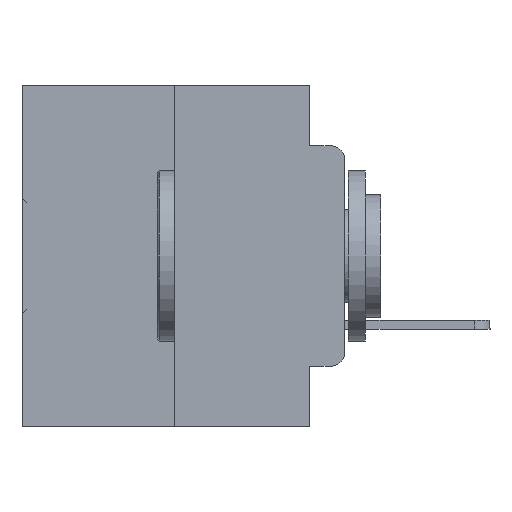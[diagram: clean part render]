
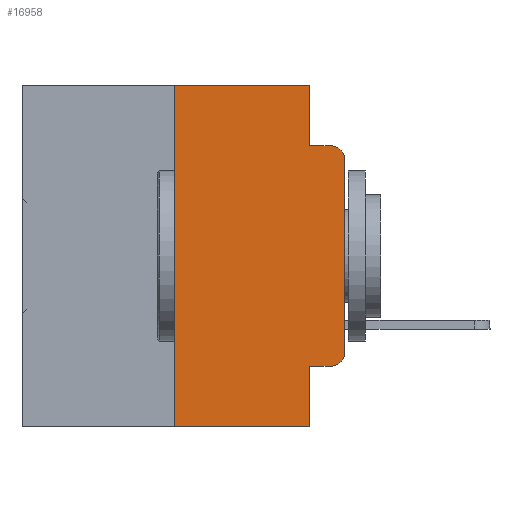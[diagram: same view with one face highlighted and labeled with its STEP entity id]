
A CAD part, left-side view. The second image highlights one B-rep face of the part: STEP entity #16958.
In plain terms, the highlighted planar face has unit normal (-1, 0, 0).
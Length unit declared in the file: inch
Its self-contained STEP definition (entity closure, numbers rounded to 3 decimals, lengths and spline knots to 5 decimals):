
#88 = CARTESIAN_POINT ( 'NONE',  ( 0., 0.473, 0. ) ) ;
#528 = VECTOR ( 'NONE', #10998, 39.37008 ) ;
#1633 = ORIENTED_EDGE ( 'NONE', *, *, #26213, .T. ) ;
#2574 = CARTESIAN_POINT ( 'NONE',  ( 0., 0., 0. ) ) ;
#2675 = CARTESIAN_POINT ( 'NONE',  ( 0., 0.051, -0.0885 ) ) ;
#2806 = ORIENTED_EDGE ( 'NONE', *, *, #7347, .F. ) ;
#3022 = FACE_OUTER_BOUND ( 'NONE', #13383, .T. ) ;
#3646 = VERTEX_POINT ( 'NONE', #28093 ) ;
#3757 = CARTESIAN_POINT ( 'NONE',  ( 0., 0.02, -0.0885 ) ) ;
#3817 = CARTESIAN_POINT ( 'NONE',  ( 0., 0.473, -0.5 ) ) ;
#3946 = VECTOR ( 'NONE', #22763, 39.37008 ) ;
#4187 = CARTESIAN_POINT ( 'NONE',  ( 0., 0.051, -0.5 ) ) ;
#4523 = DIRECTION ( 'NONE',  ( 0., 0., -1. ) ) ;
#4942 = CARTESIAN_POINT ( 'NONE',  ( 0., 0.02, -0.1085 ) ) ;
#4946 = CARTESIAN_POINT ( 'NONE',  ( 0., 0., -0.3915 ) ) ;
#5118 = DIRECTION ( 'NONE',  ( -1., 0., 0. ) ) ;
#5797 = EDGE_CURVE ( 'NONE', #19942, #8753, #29678, .T. ) ;
#6338 = VECTOR ( 'NONE', #9914, 39.37008 ) ;
#6473 = LINE ( 'NONE', #30298, #33679 ) ;
#7347 = EDGE_CURVE ( 'NONE', #3646, #16407, #23552, .T. ) ;
#7586 = AXIS2_PLACEMENT_3D ( 'NONE', #88, #24065, #20629 ) ;
#7751 = VERTEX_POINT ( 'NONE', #21239 ) ;
#7852 = VERTEX_POINT ( 'NONE', #22254 ) ;
#8035 = VERTEX_POINT ( 'NONE', #30872 ) ;
#8376 = VECTOR ( 'NONE', #26311, 39.37008 ) ;
#8753 = VERTEX_POINT ( 'NONE', #3757 ) ;
#9299 = ORIENTED_EDGE ( 'NONE', *, *, #20120, .T. ) ;
#9914 = DIRECTION ( 'NONE',  ( 0., -1., 0. ) ) ;
#10444 = ORIENTED_EDGE ( 'NONE', *, *, #15685, .F. ) ;
#10702 = ORIENTED_EDGE ( 'NONE', *, *, #32556, .F. ) ;
#10776 = CARTESIAN_POINT ( 'NONE',  ( 0., 0.02, -0.3915 ) ) ;
#10998 = DIRECTION ( 'NONE',  ( 0., 0., 1. ) ) ;
#11636 = EDGE_CURVE ( 'NONE', #8035, #8753, #13360, .T. ) ;
#11805 = VECTOR ( 'NONE', #33107, 39.37008 ) ;
#11986 = ORIENTED_EDGE ( 'NONE', *, *, #29588, .T. ) ;
#12225 = VERTEX_POINT ( 'NONE', #12378 ) ;
#12378 = CARTESIAN_POINT ( 'NONE',  ( 0., 0.051, 0. ) ) ;
#13260 = EDGE_CURVE ( 'NONE', #12225, #8035, #17118, .T. ) ;
#13360 = LINE ( 'NONE', #2675, #8376 ) ;
#13383 = EDGE_LOOP ( 'NONE', ( #1633, #26223, #28146, #19337, #10444, #10702, #11986, #2806, #9299, #28626 ) ) ;
#13938 = LINE ( 'NONE', #24482, #11805 ) ;
#14230 = VERTEX_POINT ( 'NONE', #4946 ) ;
#14445 = EDGE_CURVE ( 'NONE', #7751, #14230, #23313, .T. ) ;
#14519 = AXIS2_PLACEMENT_3D ( 'NONE', #10776, #31862, #18738 ) ;
#15441 = CARTESIAN_POINT ( 'NONE',  ( 0., 0.051, 0. ) ) ;
#15685 = EDGE_CURVE ( 'NONE', #7852, #12225, #20810, .T. ) ;
#15988 = CARTESIAN_POINT ( 'NONE',  ( 0., 0.25, -0.5 ) ) ;
#16407 = VERTEX_POINT ( 'NONE', #4187 ) ;
#16473 = DIRECTION ( 'NONE',  ( 0., -1., 0. ) ) ;
#16958 = ADVANCED_FACE ( 'NONE', ( #3022 ), #20792, .F. ) ;
#17118 = LINE ( 'NONE', #25568, #18944 ) ;
#18398 = DIRECTION ( 'NONE',  ( 0., 0., -1. ) ) ;
#18738 = DIRECTION ( 'NONE',  ( 0., 0., -1. ) ) ;
#18944 = VECTOR ( 'NONE', #4523, 39.37008 ) ;
#19337 = ORIENTED_EDGE ( 'NONE', *, *, #13260, .F. ) ;
#19942 = VERTEX_POINT ( 'NONE', #21669 ) ;
#20120 = EDGE_CURVE ( 'NONE', #3646, #7751, #6473, .T. ) ;
#20629 = DIRECTION ( 'NONE',  ( 0., 0., -1. ) ) ;
#20792 = PLANE ( 'NONE',  #7586 ) ;
#20810 = LINE ( 'NONE', #33593, #6338 ) ;
#21239 = CARTESIAN_POINT ( 'NONE',  ( 0., 0.02, -0.4115 ) ) ;
#21669 = CARTESIAN_POINT ( 'NONE',  ( 0., 0., -0.1085 ) ) ;
#22254 = CARTESIAN_POINT ( 'NONE',  ( 0., 0.25, 0. ) ) ;
#22763 = DIRECTION ( 'NONE',  ( 0., -1., 0. ) ) ;
#23313 = CIRCLE ( 'NONE', #14519, 0.02 ) ;
#23552 = LINE ( 'NONE', #15441, #30785 ) ;
#23625 = LINE ( 'NONE', #2574, #528 ) ;
#23908 = DIRECTION ( 'NONE',  ( 0., 0., -1. ) ) ;
#24065 = DIRECTION ( 'NONE',  ( 1., 0., 0. ) ) ;
#24482 = CARTESIAN_POINT ( 'NONE',  ( 0., 0.25, 0. ) ) ;
#25568 = CARTESIAN_POINT ( 'NONE',  ( 0., 0.051, 0. ) ) ;
#26213 = EDGE_CURVE ( 'NONE', #14230, #19942, #23625, .T. ) ;
#26223 = ORIENTED_EDGE ( 'NONE', *, *, #5797, .T. ) ;
#26311 = DIRECTION ( 'NONE',  ( 0., -1., 0. ) ) ;
#26374 = AXIS2_PLACEMENT_3D ( 'NONE', #4942, #5118, #18398 ) ;
#26632 = VERTEX_POINT ( 'NONE', #15988 ) ;
#28093 = CARTESIAN_POINT ( 'NONE',  ( 0., 0.051, -0.4115 ) ) ;
#28146 = ORIENTED_EDGE ( 'NONE', *, *, #11636, .F. ) ;
#28626 = ORIENTED_EDGE ( 'NONE', *, *, #14445, .T. ) ;
#29588 = EDGE_CURVE ( 'NONE', #26632, #16407, #29869, .T. ) ;
#29678 = CIRCLE ( 'NONE', #26374, 0.02 ) ;
#29869 = LINE ( 'NONE', #3817, #3946 ) ;
#30298 = CARTESIAN_POINT ( 'NONE',  ( 0., 0.051, -0.4115 ) ) ;
#30785 = VECTOR ( 'NONE', #23908, 39.37008 ) ;
#30872 = CARTESIAN_POINT ( 'NONE',  ( 0., 0.051, -0.0885 ) ) ;
#31862 = DIRECTION ( 'NONE',  ( -1., 0., 0. ) ) ;
#32556 = EDGE_CURVE ( 'NONE', #26632, #7852, #13938, .T. ) ;
#33107 = DIRECTION ( 'NONE',  ( 0., 0., 1. ) ) ;
#33593 = CARTESIAN_POINT ( 'NONE',  ( 0., 0.473, 0. ) ) ;
#33679 = VECTOR ( 'NONE', #16473, 39.37008 ) ;
